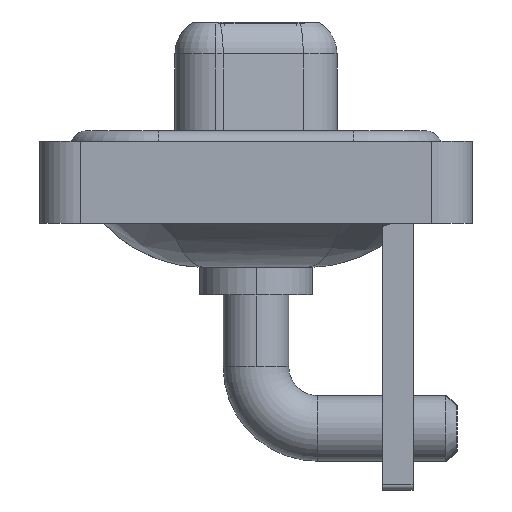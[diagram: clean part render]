
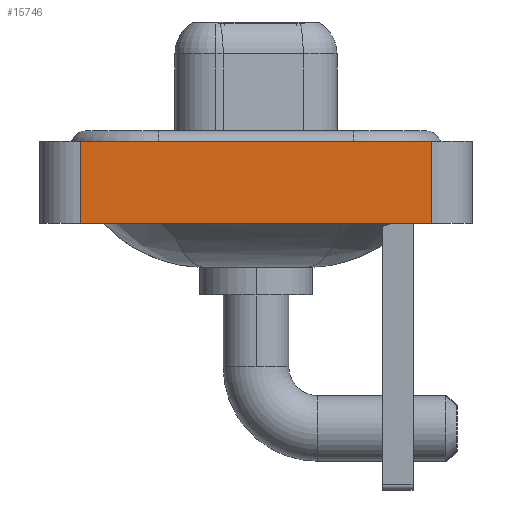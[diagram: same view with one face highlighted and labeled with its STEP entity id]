
A CAD part, left-side view. The second image highlights one B-rep face of the part: STEP entity #15746.
In plain terms, the highlighted planar face has unit normal (-1, 0, 0).
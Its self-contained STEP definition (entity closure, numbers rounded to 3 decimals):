
#120 = CARTESIAN_POINT ( 'NONE',  ( -7.25, -8.55, 0.4 ) ) ;
#1253 = DIRECTION ( 'NONE',  ( 0., -1., 0. ) ) ;
#1445 = DIRECTION ( 'NONE',  ( 0., 0., 1. ) ) ;
#2014 = EDGE_CURVE ( 'NONE', #13075, #17342, #15226, .T. ) ;
#2032 = ORIENTED_EDGE ( 'NONE', *, *, #4029, .F. ) ;
#2491 = CARTESIAN_POINT ( 'NONE',  ( -7.25, 8.55, -3.6 ) ) ;
#2626 = CARTESIAN_POINT ( 'NONE',  ( -7.25, -8.55, -3.6 ) ) ;
#2740 = VECTOR ( 'NONE', #1253, 1000. ) ;
#3834 = LINE ( 'NONE', #16097, #13456 ) ;
#4029 = EDGE_CURVE ( 'NONE', #17342, #5272, #16856, .T. ) ;
#4071 = AXIS2_PLACEMENT_3D ( 'NONE', #2626, #12367, #1445 ) ;
#4565 = VECTOR ( 'NONE', #6820, 1000. ) ;
#5272 = VERTEX_POINT ( 'NONE', #120 ) ;
#5756 = VERTEX_POINT ( 'NONE', #15574 ) ;
#5968 = VECTOR ( 'NONE', #7352, 1000. ) ;
#6501 = EDGE_CURVE ( 'NONE', #5756, #5272, #3834, .T. ) ;
#6820 = DIRECTION ( 'NONE',  ( 0., 0., 1. ) ) ;
#7071 = CARTESIAN_POINT ( 'NONE',  ( -7.25, 8.55, -3.6 ) ) ;
#7352 = DIRECTION ( 'NONE',  ( 0., -1., 0. ) ) ;
#7944 = DIRECTION ( 'NONE',  ( 0., 0., 1. ) ) ;
#8132 = LINE ( 'NONE', #9222, #2740 ) ;
#8314 = PLANE ( 'NONE',  #4071 ) ;
#9222 = CARTESIAN_POINT ( 'NONE',  ( -7.25, -8.55, -3.6 ) ) ;
#10219 = ORIENTED_EDGE ( 'NONE', *, *, #10857, .T. ) ;
#10248 = CARTESIAN_POINT ( 'NONE',  ( -7.25, 8.55, 0.4 ) ) ;
#10857 = EDGE_CURVE ( 'NONE', #13075, #5756, #8132, .T. ) ;
#10888 = EDGE_LOOP ( 'NONE', ( #14123, #2032, #15274, #10219 ) ) ;
#11486 = CARTESIAN_POINT ( 'NONE',  ( -7.25, -8.55, 0.4 ) ) ;
#12367 = DIRECTION ( 'NONE',  ( -1., 0., 0. ) ) ;
#13075 = VERTEX_POINT ( 'NONE', #2491 ) ;
#13456 = VECTOR ( 'NONE', #7944, 1000. ) ;
#13705 = FACE_OUTER_BOUND ( 'NONE', #10888, .T. ) ;
#14123 = ORIENTED_EDGE ( 'NONE', *, *, #6501, .T. ) ;
#15226 = LINE ( 'NONE', #7071, #4565 ) ;
#15274 = ORIENTED_EDGE ( 'NONE', *, *, #2014, .F. ) ;
#15574 = CARTESIAN_POINT ( 'NONE',  ( -7.25, -8.55, -3.6 ) ) ;
#15746 = ADVANCED_FACE ( 'NONE', ( #13705 ), #8314, .T. ) ;
#16097 = CARTESIAN_POINT ( 'NONE',  ( -7.25, -8.55, -3.6 ) ) ;
#16856 = LINE ( 'NONE', #11486, #5968 ) ;
#17342 = VERTEX_POINT ( 'NONE', #10248 ) ;
